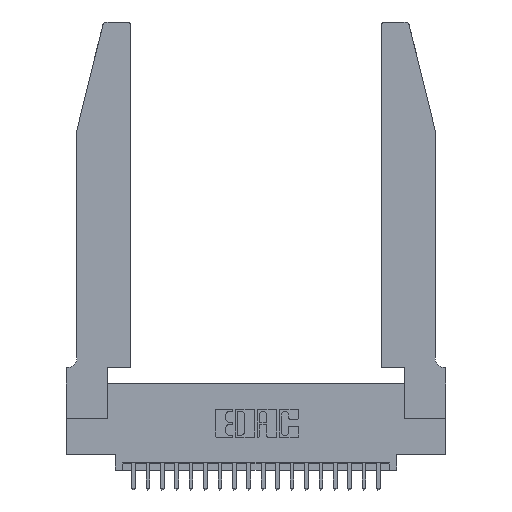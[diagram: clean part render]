
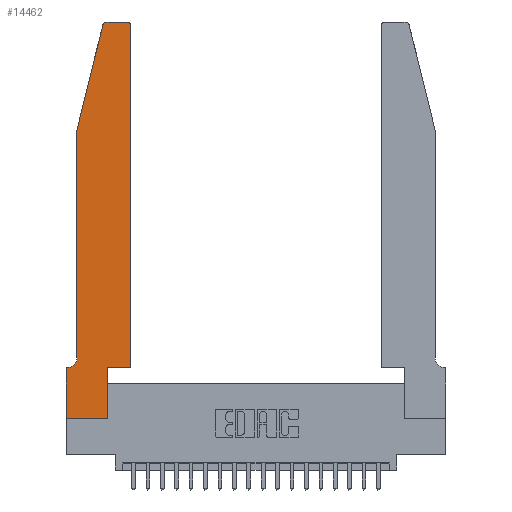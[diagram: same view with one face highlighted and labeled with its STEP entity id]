
A CAD part, top view. The second image highlights one B-rep face of the part: STEP entity #14462.
In plain terms, the highlighted planar face has unit normal (0, 0, 1).
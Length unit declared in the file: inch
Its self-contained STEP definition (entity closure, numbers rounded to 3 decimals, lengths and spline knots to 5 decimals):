
#60 = VERTEX_POINT ( 'NONE', #9910 ) ;
#241 = DIRECTION ( 'NONE',  ( 1., 0., 0. ) ) ;
#595 = DIRECTION ( 'NONE',  ( -1., 0., 0. ) ) ;
#693 = EDGE_CURVE ( 'NONE', #1714, #21747, #818, .T. ) ;
#777 = LINE ( 'NONE', #13933, #1062 ) ;
#818 = LINE ( 'NONE', #7304, #8665 ) ;
#1062 = VECTOR ( 'NONE', #241, 39.37008 ) ;
#1148 = ORIENTED_EDGE ( 'NONE', *, *, #12179, .T. ) ;
#1160 = LINE ( 'NONE', #2507, #20799 ) ;
#1206 = ORIENTED_EDGE ( 'NONE', *, *, #10197, .T. ) ;
#1550 = CIRCLE ( 'NONE', #16048, 0.03 ) ;
#1581 = CARTESIAN_POINT ( 'NONE',  ( 0.284, 2.75, 0.37 ) ) ;
#1714 = VERTEX_POINT ( 'NONE', #18673 ) ;
#1786 = DIRECTION ( 'NONE',  ( 0., 0., 1. ) ) ;
#1926 = DIRECTION ( 'NONE',  ( 0., 1., 0. ) ) ;
#2263 = EDGE_CURVE ( 'NONE', #11331, #3305, #17688, .T. ) ;
#2479 = ORIENTED_EDGE ( 'NONE', *, *, #3584, .T. ) ;
#2507 = CARTESIAN_POINT ( 'NONE',  ( 0., 0., 0.37 ) ) ;
#2649 = CARTESIAN_POINT ( 'NONE',  ( 0.2865, 0., 0.37 ) ) ;
#2820 = VERTEX_POINT ( 'NONE', #20661 ) ;
#2860 = EDGE_CURVE ( 'NONE', #60, #1714, #1550, .T. ) ;
#3264 = DIRECTION ( 'NONE',  ( -1., 0., 0. ) ) ;
#3293 = CARTESIAN_POINT ( 'NONE',  ( 0.0055, 0.42, 0.37 ) ) ;
#3305 = VERTEX_POINT ( 'NONE', #15246 ) ;
#3576 = CARTESIAN_POINT ( 'NONE',  ( 0.4505, 0.35, 0.37 ) ) ;
#3584 = EDGE_CURVE ( 'NONE', #12743, #9116, #17381, .T. ) ;
#3598 = DIRECTION ( 'NONE',  ( 0., 0., -1. ) ) ;
#4352 = FACE_OUTER_BOUND ( 'NONE', #12677, .T. ) ;
#4416 = CIRCLE ( 'NONE', #11543, 0.07 ) ;
#4530 = CARTESIAN_POINT ( 'NONE',  ( 0., 0.35, 0.37 ) ) ;
#4698 = DIRECTION ( 'NONE',  ( 0., -1., 0. ) ) ;
#5165 = CARTESIAN_POINT ( 'NONE',  ( 0.0755, 0.35, 0.37 ) ) ;
#5342 = DIRECTION ( 'NONE',  ( -1., 0., 0. ) ) ;
#5554 = VECTOR ( 'NONE', #9704, 39.37008 ) ;
#5589 = ORIENTED_EDGE ( 'NONE', *, *, #2860, .T. ) ;
#5838 = AXIS2_PLACEMENT_3D ( 'NONE', #17479, #1786, #8797 ) ;
#5942 = AXIS2_PLACEMENT_3D ( 'NONE', #19280, #12495, #7482 ) ;
#6103 = LINE ( 'NONE', #19616, #16553 ) ;
#6741 = EDGE_CURVE ( 'NONE', #11596, #12743, #13285, .T. ) ;
#6825 = CARTESIAN_POINT ( 'NONE',  ( 0.0755, 0.42, 0.37 ) ) ;
#6829 = CARTESIAN_POINT ( 'NONE',  ( 0.4205, 2.72, 0.37 ) ) ;
#7304 = CARTESIAN_POINT ( 'NONE',  ( 0.2605, 2.75, 0.37 ) ) ;
#7482 = DIRECTION ( 'NONE',  ( 1., 0., 0. ) ) ;
#7872 = EDGE_CURVE ( 'NONE', #2820, #11331, #10083, .T. ) ;
#8429 = ORIENTED_EDGE ( 'NONE', *, *, #13757, .T. ) ;
#8665 = VECTOR ( 'NONE', #595, 39.37008 ) ;
#8797 = DIRECTION ( 'NONE',  ( 1., 0., 0. ) ) ;
#9116 = VERTEX_POINT ( 'NONE', #6825 ) ;
#9262 = VECTOR ( 'NONE', #14047, 39.37008 ) ;
#9309 = DIRECTION ( 'NONE',  ( 1., 0., 0. ) ) ;
#9704 = DIRECTION ( 'NONE',  ( 0., -1., 0. ) ) ;
#9910 = CARTESIAN_POINT ( 'NONE',  ( 0.4505, 2.72, 0.37 ) ) ;
#10040 = VECTOR ( 'NONE', #1926, 39.37008 ) ;
#10083 = LINE ( 'NONE', #5165, #19216 ) ;
#10197 = EDGE_CURVE ( 'NONE', #15281, #11066, #777, .T. ) ;
#11066 = VERTEX_POINT ( 'NONE', #18455 ) ;
#11331 = VERTEX_POINT ( 'NONE', #4530 ) ;
#11543 = AXIS2_PLACEMENT_3D ( 'NONE', #3293, #3598, #5342 ) ;
#11596 = VERTEX_POINT ( 'NONE', #15038 ) ;
#11629 = CARTESIAN_POINT ( 'NONE',  ( 0.0755, 2., 0.37 ) ) ;
#12179 = EDGE_CURVE ( 'NONE', #21747, #11596, #20060, .T. ) ;
#12345 = EDGE_CURVE ( 'NONE', #9116, #2820, #4416, .T. ) ;
#12495 = DIRECTION ( 'NONE',  ( 0., 0., 1. ) ) ;
#12677 = EDGE_LOOP ( 'NONE', ( #14810, #1148, #17436, #2479, #13409, #18066, #13684, #8429, #13365, #1206, #16975, #5589 ) ) ;
#12743 = VERTEX_POINT ( 'NONE', #21162 ) ;
#13285 = LINE ( 'NONE', #18637, #9262 ) ;
#13365 = ORIENTED_EDGE ( 'NONE', *, *, #17978, .T. ) ;
#13409 = ORIENTED_EDGE ( 'NONE', *, *, #12345, .T. ) ;
#13684 = ORIENTED_EDGE ( 'NONE', *, *, #2263, .T. ) ;
#13757 = EDGE_CURVE ( 'NONE', #3305, #15834, #1160, .T. ) ;
#13933 = CARTESIAN_POINT ( 'NONE',  ( 0.4505, 0.35, 0.37 ) ) ;
#14047 = DIRECTION ( 'NONE',  ( -0.239, -0.971, 0. ) ) ;
#14291 = DIRECTION ( 'NONE',  ( 0., 1., 0. ) ) ;
#14462 = ADVANCED_FACE ( 'NONE', ( #4352 ), #20725, .T. ) ;
#14468 = EDGE_CURVE ( 'NONE', #11066, #60, #18626, .T. ) ;
#14810 = ORIENTED_EDGE ( 'NONE', *, *, #693, .T. ) ;
#14819 = CARTESIAN_POINT ( 'NONE',  ( 0., 0., 0.37 ) ) ;
#15038 = CARTESIAN_POINT ( 'NONE',  ( 0.25487, 2.72718, 0.37 ) ) ;
#15246 = CARTESIAN_POINT ( 'NONE',  ( 0., 0., 0.37 ) ) ;
#15281 = VERTEX_POINT ( 'NONE', #17927 ) ;
#15834 = VERTEX_POINT ( 'NONE', #2649 ) ;
#16048 = AXIS2_PLACEMENT_3D ( 'NONE', #6829, #20349, #22218 ) ;
#16553 = VECTOR ( 'NONE', #14291, 39.37008 ) ;
#16975 = ORIENTED_EDGE ( 'NONE', *, *, #14468, .T. ) ;
#17381 = LINE ( 'NONE', #11629, #5554 ) ;
#17436 = ORIENTED_EDGE ( 'NONE', *, *, #6741, .T. ) ;
#17479 = CARTESIAN_POINT ( 'NONE',  ( 0., 0.35, 0.37 ) ) ;
#17688 = LINE ( 'NONE', #14819, #20113 ) ;
#17927 = CARTESIAN_POINT ( 'NONE',  ( 0.2865, 0.35, 0.37 ) ) ;
#17978 = EDGE_CURVE ( 'NONE', #15834, #15281, #6103, .T. ) ;
#18066 = ORIENTED_EDGE ( 'NONE', *, *, #7872, .T. ) ;
#18455 = CARTESIAN_POINT ( 'NONE',  ( 0.4505, 0.35, 0.37 ) ) ;
#18626 = LINE ( 'NONE', #3576, #10040 ) ;
#18637 = CARTESIAN_POINT ( 'NONE',  ( 0.0755, 2., 0.37 ) ) ;
#18673 = CARTESIAN_POINT ( 'NONE',  ( 0.4205, 2.75, 0.37 ) ) ;
#19216 = VECTOR ( 'NONE', #3264, 39.37008 ) ;
#19280 = CARTESIAN_POINT ( 'NONE',  ( 0.284, 2.72, 0.37 ) ) ;
#19616 = CARTESIAN_POINT ( 'NONE',  ( 0.2865, 0.35, 0.37 ) ) ;
#20060 = CIRCLE ( 'NONE', #5942, 0.03 ) ;
#20113 = VECTOR ( 'NONE', #4698, 39.37008 ) ;
#20349 = DIRECTION ( 'NONE',  ( 0., 0., 1. ) ) ;
#20661 = CARTESIAN_POINT ( 'NONE',  ( 0.0055, 0.35, 0.37 ) ) ;
#20725 = PLANE ( 'NONE',  #5838 ) ;
#20799 = VECTOR ( 'NONE', #9309, 39.37008 ) ;
#21162 = CARTESIAN_POINT ( 'NONE',  ( 0.0755, 2., 0.37 ) ) ;
#21747 = VERTEX_POINT ( 'NONE', #1581 ) ;
#22218 = DIRECTION ( 'NONE',  ( 1., 0., 0. ) ) ;
